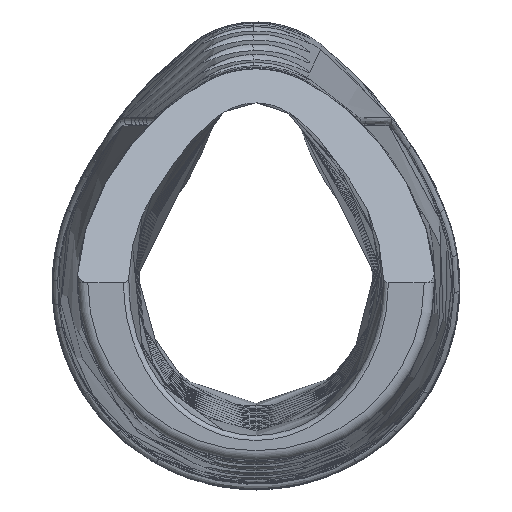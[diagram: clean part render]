
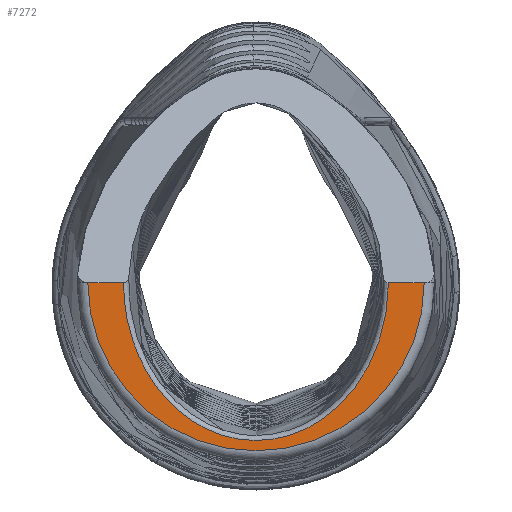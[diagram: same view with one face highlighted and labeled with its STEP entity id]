
A CAD part, top view. The second image highlights one B-rep face of the part: STEP entity #7272.
In plain terms, the highlighted planar face has unit normal (0, 0, 1).
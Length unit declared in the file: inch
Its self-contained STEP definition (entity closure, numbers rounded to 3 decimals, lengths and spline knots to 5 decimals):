
#1028 = CARTESIAN_POINT ( 'NONE',  ( -0.40222, -0.60908, 10.25 ) ) ;
#1232 = CARTESIAN_POINT ( 'NONE',  ( -0.34894, -0.65405, 10.25 ) ) ;
#1242 = B_SPLINE_CURVE_WITH_KNOTS ( 'NONE', 3,
 ( #4353, #33462, #39712, #7261, #20374, #39300, #20781, #19962, #36590, #29741, #4555, #26823, #32856, #39504, #17243, #10590, #7878, #32646, #4964, #4150, #29942, #16831, #17651, #23707, #17447, #36383, #23497, #7469, #1845, #29536, #30353, #1439, #4757, #14327, #14119, #20575, #14531, #1232, #38879, #1028, #33260, #30144, #1643, #11205, #13912, #13705, #26409, #39090, #23289, #35969, #10795, #36178, #31528, #31727 ),
 .UNSPECIFIED., .F., .F.,
 ( 4, 2, 2, 2, 2, 2, 2, 2, 2, 2, 2, 2, 2, 2, 2, 2, 2, 2, 2, 2, 2, 2, 2, 2, 2, 2, 4 ),
 ( 0.03089, 0.03269, 0.03449, 0.0381, 0.0399, 0.04171, 0.04351, 0.04531, 0.04892, 0.05072, 0.05253, 0.05433, 0.05523, 0.05613, 0.05974, 0.06155, 0.06335, 0.06696, 0.06876, 0.07056, 0.07237, 0.07417, 0.07778, 0.07958, 0.08138, 0.08499, 0.0886 ),
 .UNSPECIFIED. ) ;
#1439 = CARTESIAN_POINT ( 'NONE',  ( -0.09571, -0.76663, 10.25 ) ) ;
#1482 = DIRECTION ( 'NONE',  ( -1., 0., 0. ) ) ;
#1536 = EDGE_CURVE ( 'NONE', #7751, #21471, #27101, .T. ) ;
#1643 = CARTESIAN_POINT ( 'NONE',  ( -0.4661, -0.54048, 10.25 ) ) ;
#1845 = CARTESIAN_POINT ( 'NONE',  ( 0.04531, -0.77473, 10.25 ) ) ;
#3910 = CARTESIAN_POINT ( 'NONE',  ( -0.64987, -0.00141, 10.25 ) ) ;
#4150 = CARTESIAN_POINT ( 'NONE',  ( 0.3076, -0.68287, 10.25 ) ) ;
#4353 = CARTESIAN_POINT ( 'NONE',  ( 0.64987, -0.00141, 10.25 ) ) ;
#4555 = CARTESIAN_POINT ( 'NONE',  ( 0.56402, -0.38566, 10.25 ) ) ;
#4757 = CARTESIAN_POINT ( 'NONE',  ( -0.11858, -0.76206, 10.25 ) ) ;
#4964 = CARTESIAN_POINT ( 'NONE',  ( 0.34614, -0.65617, 10.25 ) ) ;
#5034 = DIRECTION ( 'NONE',  ( -1., 0., 0. ) ) ;
#5841 = CARTESIAN_POINT ( 'NONE',  ( 0.64987, -0.00141, 10.25 ) ) ;
#6248 = PLANE ( 'NONE',  #7621 ) ;
#7009 = ORIENTED_EDGE ( 'NONE', *, *, #31932, .T. ) ;
#7261 = CARTESIAN_POINT ( 'NONE',  ( 0.64527, -0.09496, 10.25 ) ) ;
#7272 = ADVANCED_FACE ( 'NONE', ( #28120 ), #6248, .F. ) ;
#7469 = CARTESIAN_POINT ( 'NONE',  ( 0.09153, -0.76882, 10.25 ) ) ;
#7621 = AXIS2_PLACEMENT_3D ( 'NONE', #25206, #28526, #37673 ) ;
#7751 = VERTEX_POINT ( 'NONE', #29281 ) ;
#7878 = CARTESIAN_POINT ( 'NONE',  ( 0.41777, -0.59575, 10.25 ) ) ;
#7956 = CARTESIAN_POINT ( 'NONE',  ( 0., -0.00141, 10.25 ) ) ;
#9332 = VERTEX_POINT ( 'NONE', #3910 ) ;
#10498 = CARTESIAN_POINT ( 'NONE',  ( -0.825, -0.00141, 10.25 ) ) ;
#10590 = CARTESIAN_POINT ( 'NONE',  ( 0.44959, -0.56171, 10.25 ) ) ;
#10795 = CARTESIAN_POINT ( 'NONE',  ( -0.63204, -0.1862, 10.25 ) ) ;
#10838 = DIRECTION ( 'NONE',  ( 0., 0., 1. ) ) ;
#11205 = CARTESIAN_POINT ( 'NONE',  ( -0.50844, -0.48511, 10.25 ) ) ;
#12455 = CARTESIAN_POINT ( 'NONE',  ( 0., -0.00141, 10.25 ) ) ;
#13336 = CIRCLE ( 'NONE', #40577, 0.825 ) ;
#13705 = CARTESIAN_POINT ( 'NONE',  ( -0.56464, -0.38435, 10.25 ) ) ;
#13912 = CARTESIAN_POINT ( 'NONE',  ( -0.53294, -0.446, 10.25 ) ) ;
#14119 = CARTESIAN_POINT ( 'NONE',  ( -0.22892, -0.727, 10.25 ) ) ;
#14327 = CARTESIAN_POINT ( 'NONE',  ( -0.18586, -0.74427, 10.25 ) ) ;
#14531 = CARTESIAN_POINT ( 'NONE',  ( -0.31082, -0.68079, 10.25 ) ) ;
#14578 = CARTESIAN_POINT ( 'NONE',  ( 0., 0., 10.25 ) ) ;
#16831 = CARTESIAN_POINT ( 'NONE',  ( 0.24669, -0.71715, 10.25 ) ) ;
#17243 = CARTESIAN_POINT ( 'NONE',  ( 0.4926, -0.50598, 10.25 ) ) ;
#17447 = CARTESIAN_POINT ( 'NONE',  ( 0.18167, -0.74386, 10.25 ) ) ;
#17651 = CARTESIAN_POINT ( 'NONE',  ( 0.22554, -0.72701, 10.25 ) ) ;
#19962 = CARTESIAN_POINT ( 'NONE',  ( 0.59981, -0.29916, 10.25 ) ) ;
#20374 = CARTESIAN_POINT ( 'NONE',  ( 0.64258, -0.11811, 10.25 ) ) ;
#20575 = CARTESIAN_POINT ( 'NONE',  ( -0.29093, -0.69319, 10.25 ) ) ;
#20781 = CARTESIAN_POINT ( 'NONE',  ( 0.62127, -0.23233, 10.25 ) ) ;
#21471 = VERTEX_POINT ( 'NONE', #5841 ) ;
#21668 = VERTEX_POINT ( 'NONE', #10498 ) ;
#23039 = ORIENTED_EDGE ( 'NONE', *, *, #37394, .T. ) ;
#23289 = CARTESIAN_POINT ( 'NONE',  ( -0.6002, -0.29806, 10.25 ) ) ;
#23497 = CARTESIAN_POINT ( 'NONE',  ( 0.14806, -0.75434, 10.25 ) ) ;
#23707 = CARTESIAN_POINT ( 'NONE',  ( 0.1928, -0.73988, 10.25 ) ) ;
#24960 = LINE ( 'NONE', #12455, #39751 ) ;
#25161 = DIRECTION ( 'NONE',  ( -1., 0., 0. ) ) ;
#25206 = CARTESIAN_POINT ( 'NONE',  ( 0., 0., 10.25 ) ) ;
#26409 = CARTESIAN_POINT ( 'NONE',  ( -0.57436, -0.3633, 10.25 ) ) ;
#26823 = CARTESIAN_POINT ( 'NONE',  ( 0.54265, -0.42702, 10.25 ) ) ;
#27101 = LINE ( 'NONE', #7956, #34966 ) ;
#28120 = FACE_OUTER_BOUND ( 'NONE', #40901, .T. ) ;
#28526 = DIRECTION ( 'NONE',  ( 0., 0., -1. ) ) ;
#29281 = CARTESIAN_POINT ( 'NONE',  ( 0.825, -0.00141, 10.25 ) ) ;
#29536 = CARTESIAN_POINT ( 'NONE',  ( -0.02547, -0.77449, 10.25 ) ) ;
#29741 = CARTESIAN_POINT ( 'NONE',  ( 0.57382, -0.36451, 10.25 ) ) ;
#29745 = EDGE_CURVE ( 'NONE', #21471, #9332, #1242, .T. ) ;
#29942 = CARTESIAN_POINT ( 'NONE',  ( 0.28772, -0.69508, 10.25 ) ) ;
#30144 = CARTESIAN_POINT ( 'NONE',  ( -0.45097, -0.55845, 10.25 ) ) ;
#30353 = CARTESIAN_POINT ( 'NONE',  ( -0.04902, -0.77286, 10.25 ) ) ;
#31528 = CARTESIAN_POINT ( 'NONE',  ( -0.6498, -0.04831, 10.25 ) ) ;
#31727 = CARTESIAN_POINT ( 'NONE',  ( -0.64987, -0.00141, 10.25 ) ) ;
#31932 = EDGE_CURVE ( 'NONE', #21668, #7751, #13336, .T. ) ;
#32646 = CARTESIAN_POINT ( 'NONE',  ( 0.36479, -0.64166, 10.25 ) ) ;
#32856 = CARTESIAN_POINT ( 'NONE',  ( 0.53108, -0.44723, 10.25 ) ) ;
#33260 = CARTESIAN_POINT ( 'NONE',  ( -0.41896, -0.59282, 10.25 ) ) ;
#33462 = CARTESIAN_POINT ( 'NONE',  ( 0.64984, -0.02477, 10.25 ) ) ;
#34154 = ORIENTED_EDGE ( 'NONE', *, *, #29745, .T. ) ;
#34966 = VECTOR ( 'NONE', #5034, 39.37008 ) ;
#35969 = CARTESIAN_POINT ( 'NONE',  ( -0.62152, -0.23134, 10.25 ) ) ;
#36178 = CARTESIAN_POINT ( 'NONE',  ( -0.64617, -0.09473, 10.25 ) ) ;
#36383 = CARTESIAN_POINT ( 'NONE',  ( 0.15931, -0.75109, 10.25 ) ) ;
#36590 = CARTESIAN_POINT ( 'NONE',  ( 0.59171, -0.3213, 10.25 ) ) ;
#37394 = EDGE_CURVE ( 'NONE', #9332, #21668, #24960, .T. ) ;
#37673 = DIRECTION ( 'NONE',  ( -1., 0., 0. ) ) ;
#38879 = CARTESIAN_POINT ( 'NONE',  ( -0.36721, -0.63969, 10.25 ) ) ;
#39090 = CARTESIAN_POINT ( 'NONE',  ( -0.59213, -0.3202, 10.25 ) ) ;
#39290 = ORIENTED_EDGE ( 'NONE', *, *, #1536, .T. ) ;
#39300 = CARTESIAN_POINT ( 'NONE',  ( 0.63187, -0.18705, 10.25 ) ) ;
#39504 = CARTESIAN_POINT ( 'NONE',  ( 0.50608, -0.48668, 10.25 ) ) ;
#39712 = CARTESIAN_POINT ( 'NONE',  ( 0.64891, -0.04831, 10.25 ) ) ;
#39751 = VECTOR ( 'NONE', #25161, 39.37008 ) ;
#40577 = AXIS2_PLACEMENT_3D ( 'NONE', #14578, #10838, #1482 ) ;
#40901 = EDGE_LOOP ( 'NONE', ( #7009, #39290, #34154, #23039 ) ) ;
